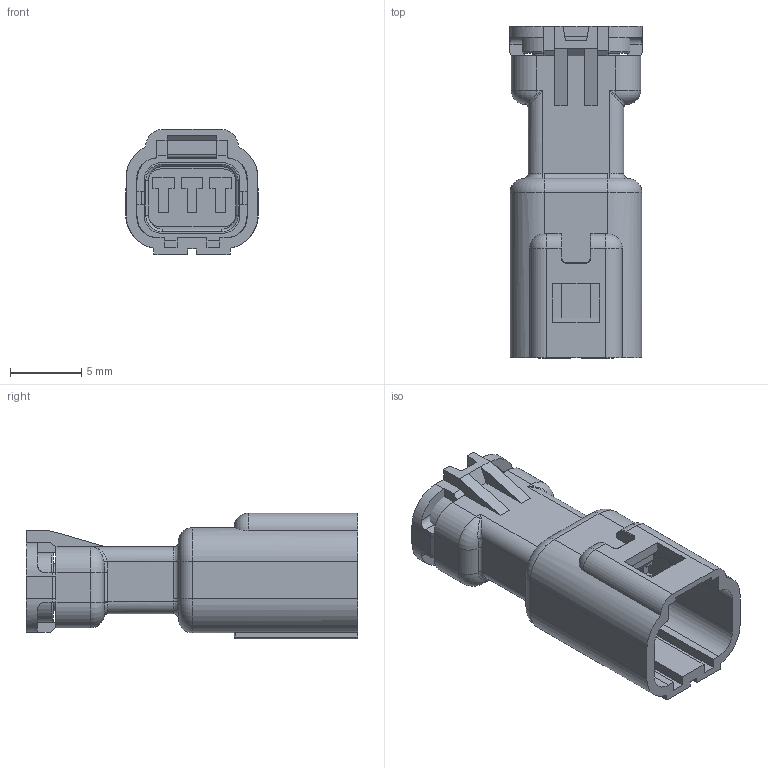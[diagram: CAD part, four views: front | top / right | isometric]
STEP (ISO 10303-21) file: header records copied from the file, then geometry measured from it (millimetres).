
FILE_DESCRIPTION (( 'STEP AP203' ), '1' );
FILE_NAME ('566-003-000-710.STEP', '2021-09-21T18:39:24', ( '' ), ( '' ), 'SwSTEP 2.0', 'SolidWorks 2020', '' );
FILE_SCHEMA (( 'CONFIG_CONTROL_DESIGN' ));
Length unit declared in the file: millimetre
Products named in the file (1): 566-003-000-710
Bounding box: 9.3 x 23.3 x 8.8 mm (x, y, z)
Volume: 722.6 mm3; surface area: 1821.7 mm2
Topology: 2 solids, 2 shells, 696 faces, 1933 edges, 1214 vertices
Faces by surface type: plane 367, cylinder 211, torus 74, bspline 24, sphere 12, cone 8
Entity records: 22882 total; most frequent: CARTESIAN_POINT 4934, ORIENTED_EDGE 3838, DIRECTION 3681, EDGE_CURVE 1919, LINE 1235, VECTOR 1235, AXIS2_PLACEMENT_3D 1223, VERTEX_POINT 1214
